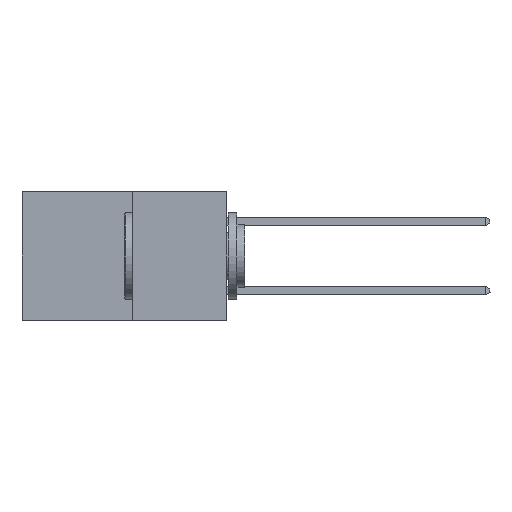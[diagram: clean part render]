
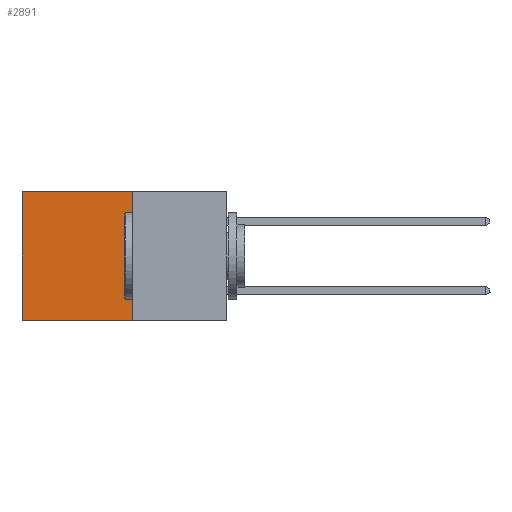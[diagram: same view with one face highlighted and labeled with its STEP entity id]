
A CAD part, left-side view. The second image highlights one B-rep face of the part: STEP entity #2891.
In plain terms, the highlighted planar face has unit normal (-1, 0, 0).
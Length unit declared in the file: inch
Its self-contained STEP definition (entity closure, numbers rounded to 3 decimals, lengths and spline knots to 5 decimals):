
#622 = CARTESIAN_POINT ( 'NONE',  ( 0.277, 0.27, 0. ) ) ;
#1641 = EDGE_CURVE ( 'NONE', #11001, #8413, #9144, .T. ) ;
#2228 = DIRECTION ( 'NONE',  ( 0., 1., 0. ) ) ;
#2246 = CARTESIAN_POINT ( 'NONE',  ( 0.277, 0.27, -0.37 ) ) ;
#2343 = VECTOR ( 'NONE', #2228, 39.37008 ) ;
#2410 = FACE_OUTER_BOUND ( 'NONE', #8661, .T. ) ;
#2464 = AXIS2_PLACEMENT_3D ( 'NONE', #3361, #2848, #2804 ) ;
#2532 = ORIENTED_EDGE ( 'NONE', *, *, #4227, .T. ) ;
#2804 = DIRECTION ( 'NONE',  ( 0., 0., -1. ) ) ;
#2848 = DIRECTION ( 'NONE',  ( 1., 0., 0. ) ) ;
#2891 = ADVANCED_FACE ( 'NONE', ( #2410 ), #3252, .F. ) ;
#3252 = PLANE ( 'NONE',  #2464 ) ;
#3339 = CARTESIAN_POINT ( 'NONE',  ( 0.277, 0.27, 0. ) ) ;
#3361 = CARTESIAN_POINT ( 'NONE',  ( 0.277, 0.27, -0.37 ) ) ;
#3417 = VECTOR ( 'NONE', #7411, 39.37008 ) ;
#3452 = DIRECTION ( 'NONE',  ( 0., 1., 0. ) ) ;
#4028 = LINE ( 'NONE', #7475, #3417 ) ;
#4227 = EDGE_CURVE ( 'NONE', #4261, #4375, #4028, .T. ) ;
#4261 = VERTEX_POINT ( 'NONE', #7264 ) ;
#4375 = VERTEX_POINT ( 'NONE', #7070 ) ;
#4731 = VECTOR ( 'NONE', #3452, 39.37008 ) ;
#5238 = ORIENTED_EDGE ( 'NONE', *, *, #1641, .F. ) ;
#5575 = EDGE_CURVE ( 'NONE', #8413, #4375, #8726, .T. ) ;
#5786 = DIRECTION ( 'NONE',  ( 0., 0., -1. ) ) ;
#6903 = LINE ( 'NONE', #3339, #4731 ) ;
#6977 = EDGE_CURVE ( 'NONE', #11001, #4261, #6903, .T. ) ;
#7070 = CARTESIAN_POINT ( 'NONE',  ( 0.277, 0.59, -0.37 ) ) ;
#7260 = CARTESIAN_POINT ( 'NONE',  ( 0.277, 0.27, -0.37 ) ) ;
#7264 = CARTESIAN_POINT ( 'NONE',  ( 0.277, 0.59, 0. ) ) ;
#7411 = DIRECTION ( 'NONE',  ( 0., 0., -1. ) ) ;
#7475 = CARTESIAN_POINT ( 'NONE',  ( 0.277, 0.59, -0.37 ) ) ;
#8018 = ORIENTED_EDGE ( 'NONE', *, *, #6977, .T. ) ;
#8413 = VERTEX_POINT ( 'NONE', #7260 ) ;
#8661 = EDGE_LOOP ( 'NONE', ( #2532, #9044, #5238, #8018 ) ) ;
#8726 = LINE ( 'NONE', #2246, #2343 ) ;
#8883 = CARTESIAN_POINT ( 'NONE',  ( 0.277, 0.27, -0.37 ) ) ;
#8902 = VECTOR ( 'NONE', #5786, 39.37008 ) ;
#9044 = ORIENTED_EDGE ( 'NONE', *, *, #5575, .F. ) ;
#9144 = LINE ( 'NONE', #8883, #8902 ) ;
#11001 = VERTEX_POINT ( 'NONE', #622 ) ;
